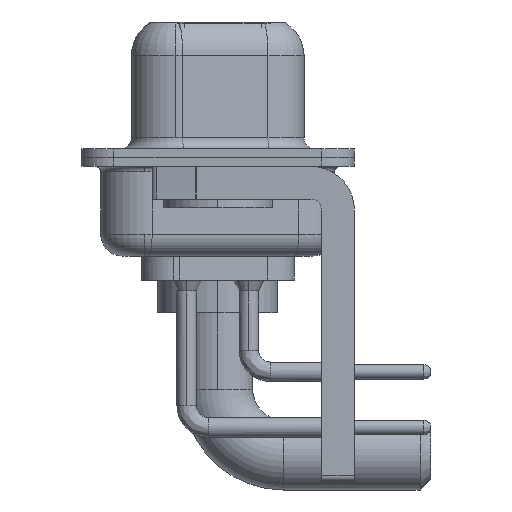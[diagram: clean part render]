
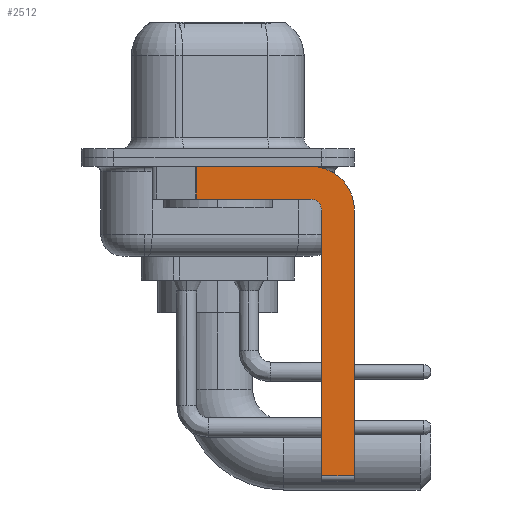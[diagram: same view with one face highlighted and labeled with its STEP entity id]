
A CAD part, left-side view. The second image highlights one B-rep face of the part: STEP entity #2512.
In plain terms, the highlighted planar face has unit normal (-1, 0, 0).
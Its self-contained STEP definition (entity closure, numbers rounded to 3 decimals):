
#1001 = LINE ( 'NONE', #18678, #9484 ) ;
#1141 = DIRECTION ( 'NONE',  ( 0., 1., 0. ) ) ;
#1318 = LINE ( 'NONE', #11701, #10375 ) ;
#1335 = CARTESIAN_POINT ( 'NONE',  ( -2.9, 0.978, -0.4 ) ) ;
#1533 = CARTESIAN_POINT ( 'NONE',  ( -2.9, -4.75, -2.4 ) ) ;
#1556 = EDGE_CURVE ( 'NONE', #8806, #12094, #14643, .T. ) ;
#1593 = LINE ( 'NONE', #4381, #18469 ) ;
#1664 = VERTEX_POINT ( 'NONE', #7525 ) ;
#1923 = CARTESIAN_POINT ( 'NONE',  ( -2.9, -4.25, -1.9 ) ) ;
#2042 = ORIENTED_EDGE ( 'NONE', *, *, #18699, .F. ) ;
#2207 = LINE ( 'NONE', #5091, #4674 ) ;
#2512 = ADVANCED_FACE ( 'NONE', ( #14303 ), #3988, .F. ) ;
#2549 = DIRECTION ( 'NONE',  ( 0., 0., -1. ) ) ;
#2944 = VERTEX_POINT ( 'NONE', #13086 ) ;
#3458 = DIRECTION ( 'NONE',  ( 0., 0., -1. ) ) ;
#3988 = PLANE ( 'NONE',  #12584 ) ;
#4381 = CARTESIAN_POINT ( 'NONE',  ( -2.9, -4.75, -14.8 ) ) ;
#4623 = EDGE_CURVE ( 'NONE', #4642, #12094, #14439, .T. ) ;
#4642 = VERTEX_POINT ( 'NONE', #1335 ) ;
#4674 = VECTOR ( 'NONE', #3458, 1000. ) ;
#5091 = CARTESIAN_POINT ( 'NONE',  ( -2.9, -6.25, -2.4 ) ) ;
#6046 = ORIENTED_EDGE ( 'NONE', *, *, #8706, .F. ) ;
#6121 = ORIENTED_EDGE ( 'NONE', *, *, #15593, .F. ) ;
#7145 = AXIS2_PLACEMENT_3D ( 'NONE', #12202, #11038, #11133 ) ;
#7525 = CARTESIAN_POINT ( 'NONE',  ( -2.9, -6.25, -2.4 ) ) ;
#7658 = EDGE_CURVE ( 'NONE', #10266, #1664, #9266, .T. ) ;
#8081 = CIRCLE ( 'NONE', #7145, 0.5 ) ;
#8495 = CARTESIAN_POINT ( 'NONE',  ( -2.9, -4.25, -1.9 ) ) ;
#8599 = VECTOR ( 'NONE', #17451, 1000. ) ;
#8659 = ORIENTED_EDGE ( 'NONE', *, *, #15074, .T. ) ;
#8706 = EDGE_CURVE ( 'NONE', #16771, #8806, #8081, .T. ) ;
#8764 = EDGE_CURVE ( 'NONE', #1664, #2944, #2207, .T. ) ;
#8806 = VERTEX_POINT ( 'NONE', #1923 ) ;
#8968 = CARTESIAN_POINT ( 'NONE',  ( -2.9, 0.978, -1.9 ) ) ;
#8977 = ORIENTED_EDGE ( 'NONE', *, *, #7658, .F. ) ;
#9266 = CIRCLE ( 'NONE', #14259, 2. ) ;
#9484 = VECTOR ( 'NONE', #17217, 1000. ) ;
#9741 = VERTEX_POINT ( 'NONE', #11453 ) ;
#9898 = CARTESIAN_POINT ( 'NONE',  ( -2.9, -4.25, -2.4 ) ) ;
#10266 = VERTEX_POINT ( 'NONE', #14347 ) ;
#10284 = DIRECTION ( 'NONE',  ( 1., 0., 0. ) ) ;
#10375 = VECTOR ( 'NONE', #15799, 1000. ) ;
#11038 = DIRECTION ( 'NONE',  ( -1., 0., 0. ) ) ;
#11133 = DIRECTION ( 'NONE',  ( 0., 0., 1. ) ) ;
#11453 = CARTESIAN_POINT ( 'NONE',  ( -2.9, -4.75, -14.55 ) ) ;
#11701 = CARTESIAN_POINT ( 'NONE',  ( -2.9, -4.25, -14.55 ) ) ;
#11945 = VECTOR ( 'NONE', #1141, 1000. ) ;
#12094 = VERTEX_POINT ( 'NONE', #8968 ) ;
#12157 = ORIENTED_EDGE ( 'NONE', *, *, #8764, .F. ) ;
#12202 = CARTESIAN_POINT ( 'NONE',  ( -2.9, -4.25, -2.4 ) ) ;
#12584 = AXIS2_PLACEMENT_3D ( 'NONE', #9898, #15869, #2549 ) ;
#12850 = DIRECTION ( 'NONE',  ( 0., 0., -1. ) ) ;
#13086 = CARTESIAN_POINT ( 'NONE',  ( -2.9, -6.25, -14.55 ) ) ;
#14259 = AXIS2_PLACEMENT_3D ( 'NONE', #14879, #10284, #12850 ) ;
#14303 = FACE_OUTER_BOUND ( 'NONE', #14783, .T. ) ;
#14347 = CARTESIAN_POINT ( 'NONE',  ( -2.9, -4.25, -0.4 ) ) ;
#14439 = LINE ( 'NONE', #19114, #8599 ) ;
#14643 = LINE ( 'NONE', #8495, #11945 ) ;
#14723 = ORIENTED_EDGE ( 'NONE', *, *, #4623, .T. ) ;
#14783 = EDGE_LOOP ( 'NONE', ( #2042, #14723, #16247, #6046, #6121, #8659, #12157, #8977 ) ) ;
#14879 = CARTESIAN_POINT ( 'NONE',  ( -2.9, -4.25, -2.4 ) ) ;
#15074 = EDGE_CURVE ( 'NONE', #9741, #2944, #1318, .T. ) ;
#15593 = EDGE_CURVE ( 'NONE', #9741, #16771, #1593, .T. ) ;
#15799 = DIRECTION ( 'NONE',  ( 0., -1., 0. ) ) ;
#15869 = DIRECTION ( 'NONE',  ( 1., 0., 0. ) ) ;
#16247 = ORIENTED_EDGE ( 'NONE', *, *, #1556, .F. ) ;
#16267 = DIRECTION ( 'NONE',  ( 0., 0., 1. ) ) ;
#16771 = VERTEX_POINT ( 'NONE', #1533 ) ;
#17217 = DIRECTION ( 'NONE',  ( 0., -1., 0. ) ) ;
#17451 = DIRECTION ( 'NONE',  ( 0., 0., -1. ) ) ;
#18469 = VECTOR ( 'NONE', #16267, 1000. ) ;
#18678 = CARTESIAN_POINT ( 'NONE',  ( -2.9, 3., -0.4 ) ) ;
#18699 = EDGE_CURVE ( 'NONE', #4642, #10266, #1001, .T. ) ;
#19114 = CARTESIAN_POINT ( 'NONE',  ( -2.9, 0.978, -1.9 ) ) ;
